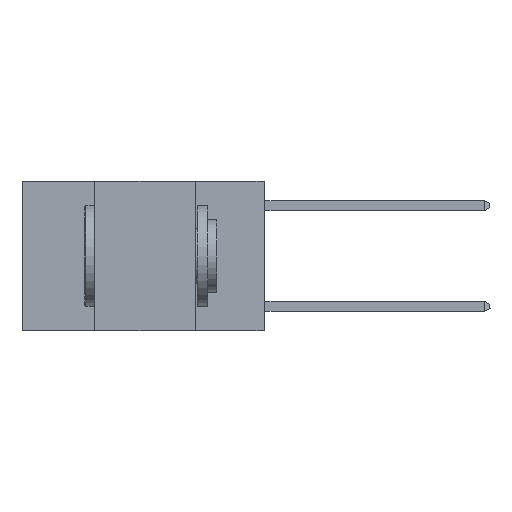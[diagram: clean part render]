
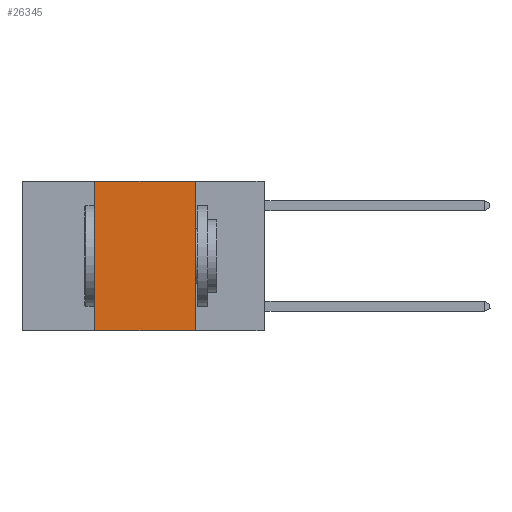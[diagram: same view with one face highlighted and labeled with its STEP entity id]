
A CAD part, left-side view. The second image highlights one B-rep face of the part: STEP entity #26345.
In plain terms, the highlighted planar face has unit normal (-1, 0, 0).
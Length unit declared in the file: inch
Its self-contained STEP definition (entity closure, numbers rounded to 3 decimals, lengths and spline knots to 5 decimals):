
#339 = CARTESIAN_POINT ( 'NONE',  ( 0., 0.17, 0. ) ) ;
#669 = LINE ( 'NONE', #26537, #17073 ) ;
#1489 = VERTEX_POINT ( 'NONE', #16266 ) ;
#2291 = DIRECTION ( 'NONE',  ( 0., -1., 0. ) ) ;
#2445 = LINE ( 'NONE', #339, #5397 ) ;
#4509 = CARTESIAN_POINT ( 'NONE',  ( 0., 0.6, 0. ) ) ;
#5397 = VECTOR ( 'NONE', #18637, 39.37008 ) ;
#5575 = CARTESIAN_POINT ( 'NONE',  ( 0., 0.42, 0. ) ) ;
#5688 = CARTESIAN_POINT ( 'NONE',  ( 0., 0.17, 0. ) ) ;
#9289 = EDGE_CURVE ( 'NONE', #24086, #15523, #669, .T. ) ;
#9447 = VECTOR ( 'NONE', #22311, 39.37008 ) ;
#9626 = AXIS2_PLACEMENT_3D ( 'NONE', #4509, #12871, #25746 ) ;
#11141 = DIRECTION ( 'NONE',  ( 0., -1., 0. ) ) ;
#11201 = ORIENTED_EDGE ( 'NONE', *, *, #13042, .F. ) ;
#11846 = VERTEX_POINT ( 'NONE', #16264 ) ;
#12410 = ORIENTED_EDGE ( 'NONE', *, *, #9289, .F. ) ;
#12498 = EDGE_CURVE ( 'NONE', #1489, #24086, #13640, .T. ) ;
#12871 = DIRECTION ( 'NONE',  ( 1., 0., 0. ) ) ;
#12893 = CARTESIAN_POINT ( 'NONE',  ( 0., 0.6, -0.37 ) ) ;
#13042 = EDGE_CURVE ( 'NONE', #15523, #11846, #2445, .T. ) ;
#13640 = LINE ( 'NONE', #22166, #9447 ) ;
#14854 = PLANE ( 'NONE',  #9626 ) ;
#15523 = VERTEX_POINT ( 'NONE', #5688 ) ;
#15800 = LINE ( 'NONE', #12893, #24957 ) ;
#16264 = CARTESIAN_POINT ( 'NONE',  ( 0., 0.17, -0.37 ) ) ;
#16266 = CARTESIAN_POINT ( 'NONE',  ( 0., 0.42, -0.37 ) ) ;
#16948 = FACE_OUTER_BOUND ( 'NONE', #26719, .T. ) ;
#17073 = VECTOR ( 'NONE', #11141, 39.37008 ) ;
#18637 = DIRECTION ( 'NONE',  ( 0., 0., -1. ) ) ;
#21156 = EDGE_CURVE ( 'NONE', #1489, #11846, #15800, .T. ) ;
#21489 = ORIENTED_EDGE ( 'NONE', *, *, #21156, .T. ) ;
#22166 = CARTESIAN_POINT ( 'NONE',  ( 0., 0.42, 0. ) ) ;
#22311 = DIRECTION ( 'NONE',  ( 0., 0., 1. ) ) ;
#24086 = VERTEX_POINT ( 'NONE', #5575 ) ;
#24957 = VECTOR ( 'NONE', #2291, 39.37008 ) ;
#25746 = DIRECTION ( 'NONE',  ( 0., 0., -1. ) ) ;
#26345 = ADVANCED_FACE ( 'NONE', ( #16948 ), #14854, .F. ) ;
#26537 = CARTESIAN_POINT ( 'NONE',  ( 0., 0.6, 0. ) ) ;
#26719 = EDGE_LOOP ( 'NONE', ( #11201, #12410, #27128, #21489 ) ) ;
#27128 = ORIENTED_EDGE ( 'NONE', *, *, #12498, .F. ) ;
